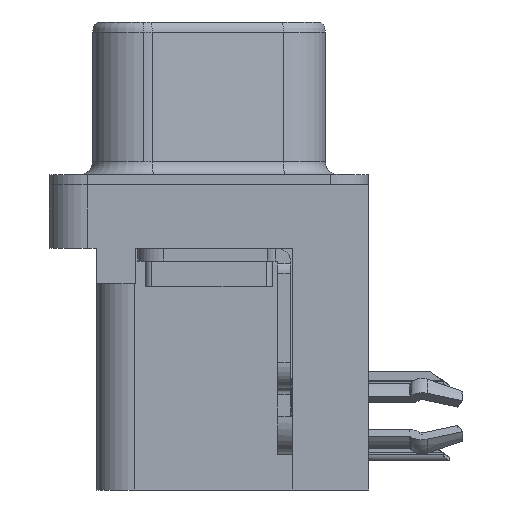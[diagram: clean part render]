
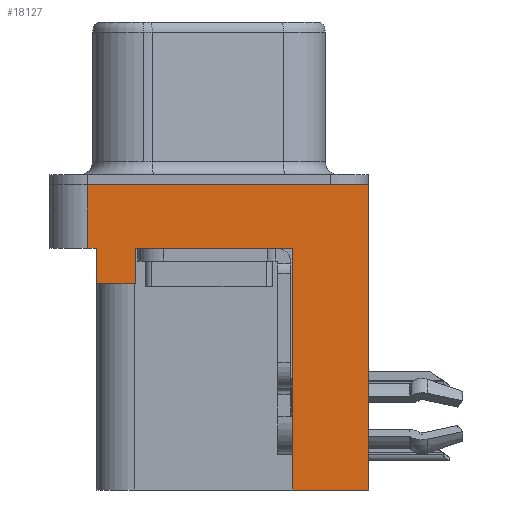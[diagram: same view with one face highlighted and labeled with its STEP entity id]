
A CAD part, left-side view. The second image highlights one B-rep face of the part: STEP entity #18127.
In plain terms, the highlighted planar face has unit normal (-1, 0, 0).
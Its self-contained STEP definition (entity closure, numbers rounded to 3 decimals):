
#13 = DIRECTION ( 'NONE',  ( 0., 0., 1. ) ) ;
#669 = ORIENTED_EDGE ( 'NONE', *, *, #14574, .T. ) ;
#1987 = DIRECTION ( 'NONE',  ( 0., 0., 1. ) ) ;
#1993 = CARTESIAN_POINT ( 'NONE',  ( -3., -6.275, 0. ) ) ;
#2100 = VECTOR ( 'NONE', #7014, 1000. ) ;
#2411 = VECTOR ( 'NONE', #1987, 1000. ) ;
#2425 = DIRECTION ( 'NONE',  ( -1., 0., 0. ) ) ;
#2466 = LINE ( 'NONE', #20650, #19101 ) ;
#2483 = LINE ( 'NONE', #22296, #19174 ) ;
#2561 = CARTESIAN_POINT ( 'NONE',  ( -3., 2.895, -3.9 ) ) ;
#3208 = EDGE_LOOP ( 'NONE', ( #13662, #22002, #7809, #16178, #9791, #669, #19405, #8094, #18007, #16226 ) ) ;
#3455 = FACE_OUTER_BOUND ( 'NONE', #3208, .T. ) ;
#3568 = VERTEX_POINT ( 'NONE', #10485 ) ;
#3581 = VERTEX_POINT ( 'NONE', #6931 ) ;
#4070 = EDGE_CURVE ( 'NONE', #20936, #3581, #19207, .T. ) ;
#4267 = CARTESIAN_POINT ( 'NONE',  ( -3., 4.775, -2.5 ) ) ;
#4696 = VECTOR ( 'NONE', #20543, 1000. ) ;
#4834 = LINE ( 'NONE', #6946, #2411 ) ;
#5721 = CARTESIAN_POINT ( 'NONE',  ( -3., -6.275, -2.5 ) ) ;
#5847 = EDGE_CURVE ( 'NONE', #20554, #16437, #4834, .T. ) ;
#6345 = DIRECTION ( 'NONE',  ( 0., -1., 0. ) ) ;
#6471 = DIRECTION ( 'NONE',  ( 0., -1., 0. ) ) ;
#6822 = EDGE_CURVE ( 'NONE', #13117, #20554, #2466, .T. ) ;
#6931 = CARTESIAN_POINT ( 'NONE',  ( -3., -3.295, -2.5 ) ) ;
#6946 = CARTESIAN_POINT ( 'NONE',  ( -3., 4.425, -3.9 ) ) ;
#7014 = DIRECTION ( 'NONE',  ( 0., 0., 1. ) ) ;
#7087 = LINE ( 'NONE', #9826, #17644 ) ;
#7809 = ORIENTED_EDGE ( 'NONE', *, *, #22121, .T. ) ;
#8094 = ORIENTED_EDGE ( 'NONE', *, *, #20013, .F. ) ;
#8734 = CARTESIAN_POINT ( 'NONE',  ( -3., 4.425, -3.9 ) ) ;
#8983 = LINE ( 'NONE', #22227, #4696 ) ;
#9503 = LINE ( 'NONE', #21191, #11152 ) ;
#9788 = AXIS2_PLACEMENT_3D ( 'NONE', #5721, #2425, #11010 ) ;
#9791 = ORIENTED_EDGE ( 'NONE', *, *, #6822, .F. ) ;
#9798 = CARTESIAN_POINT ( 'NONE',  ( -3., -6.275, -12. ) ) ;
#9826 = CARTESIAN_POINT ( 'NONE',  ( -3., -6.275, -2.5 ) ) ;
#10032 = CARTESIAN_POINT ( 'NONE',  ( -3., -6.275, -2.5 ) ) ;
#10485 = CARTESIAN_POINT ( 'NONE',  ( -3., -6.275, 0. ) ) ;
#11010 = DIRECTION ( 'NONE',  ( 0., 0., 1. ) ) ;
#11152 = VECTOR ( 'NONE', #14142, 1000. ) ;
#11285 = LINE ( 'NONE', #19016, #2100 ) ;
#11354 = EDGE_CURVE ( 'NONE', #18318, #11844, #11285, .T. ) ;
#11369 = DIRECTION ( 'NONE',  ( 0., 0., 1. ) ) ;
#11467 = CARTESIAN_POINT ( 'NONE',  ( -3., 2.895, -2.5 ) ) ;
#11844 = VERTEX_POINT ( 'NONE', #11926 ) ;
#11926 = CARTESIAN_POINT ( 'NONE',  ( -3., 4.775, 0. ) ) ;
#12723 = VERTEX_POINT ( 'NONE', #21587 ) ;
#13117 = VERTEX_POINT ( 'NONE', #19886 ) ;
#13662 = ORIENTED_EDGE ( 'NONE', *, *, #17376, .F. ) ;
#14142 = DIRECTION ( 'NONE',  ( 0., 0., 1. ) ) ;
#14574 = EDGE_CURVE ( 'NONE', #13117, #20936, #22108, .T. ) ;
#15544 = EDGE_CURVE ( 'NONE', #16617, #12723, #8983, .T. ) ;
#16178 = ORIENTED_EDGE ( 'NONE', *, *, #5847, .F. ) ;
#16207 = VECTOR ( 'NONE', #19106, 1000. ) ;
#16226 = ORIENTED_EDGE ( 'NONE', *, *, #18913, .T. ) ;
#16437 = VERTEX_POINT ( 'NONE', #17943 ) ;
#16617 = VERTEX_POINT ( 'NONE', #9798 ) ;
#17058 = VECTOR ( 'NONE', #6471, 1000. ) ;
#17376 = EDGE_CURVE ( 'NONE', #11844, #3568, #17530, .T. ) ;
#17530 = LINE ( 'NONE', #1993, #16207 ) ;
#17644 = VECTOR ( 'NONE', #6345, 1000. ) ;
#17943 = CARTESIAN_POINT ( 'NONE',  ( -3., 4.425, -2.5 ) ) ;
#18007 = ORIENTED_EDGE ( 'NONE', *, *, #15544, .F. ) ;
#18127 = ADVANCED_FACE ( 'NONE', ( #3455 ), #19525, .T. ) ;
#18318 = VERTEX_POINT ( 'NONE', #4267 ) ;
#18913 = EDGE_CURVE ( 'NONE', #16617, #3568, #9503, .T. ) ;
#19016 = CARTESIAN_POINT ( 'NONE',  ( -3., 4.775, -2.5 ) ) ;
#19101 = VECTOR ( 'NONE', #21096, 1000. ) ;
#19106 = DIRECTION ( 'NONE',  ( 0., -1., 0. ) ) ;
#19174 = VECTOR ( 'NONE', #13, 1000. ) ;
#19207 = LINE ( 'NONE', #10032, #17058 ) ;
#19405 = ORIENTED_EDGE ( 'NONE', *, *, #4070, .T. ) ;
#19525 = PLANE ( 'NONE',  #9788 ) ;
#19886 = CARTESIAN_POINT ( 'NONE',  ( -3., 2.895, -3.9 ) ) ;
#20013 = EDGE_CURVE ( 'NONE', #12723, #3581, #2483, .T. ) ;
#20543 = DIRECTION ( 'NONE',  ( 0., 1., 0. ) ) ;
#20554 = VERTEX_POINT ( 'NONE', #8734 ) ;
#20650 = CARTESIAN_POINT ( 'NONE',  ( -3., 4.425, -3.9 ) ) ;
#20753 = VECTOR ( 'NONE', #11369, 1000. ) ;
#20936 = VERTEX_POINT ( 'NONE', #11467 ) ;
#21096 = DIRECTION ( 'NONE',  ( 0., 1., 0. ) ) ;
#21191 = CARTESIAN_POINT ( 'NONE',  ( -3., -6.275, -2.5 ) ) ;
#21587 = CARTESIAN_POINT ( 'NONE',  ( -3., -3.295, -12. ) ) ;
#22002 = ORIENTED_EDGE ( 'NONE', *, *, #11354, .F. ) ;
#22108 = LINE ( 'NONE', #2561, #20753 ) ;
#22121 = EDGE_CURVE ( 'NONE', #18318, #16437, #7087, .T. ) ;
#22227 = CARTESIAN_POINT ( 'NONE',  ( -3., -3.295, -12. ) ) ;
#22296 = CARTESIAN_POINT ( 'NONE',  ( -3., -3.295, -12. ) ) ;
